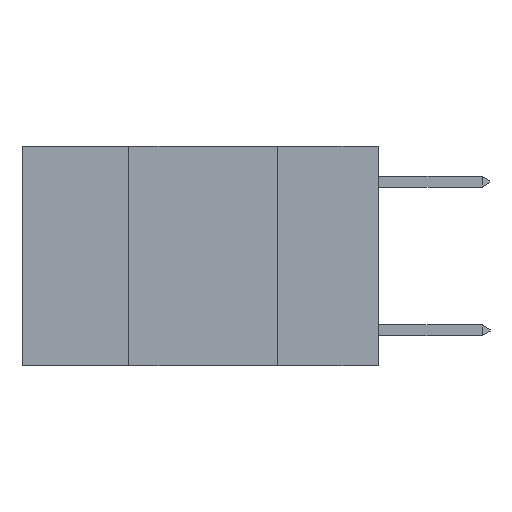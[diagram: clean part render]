
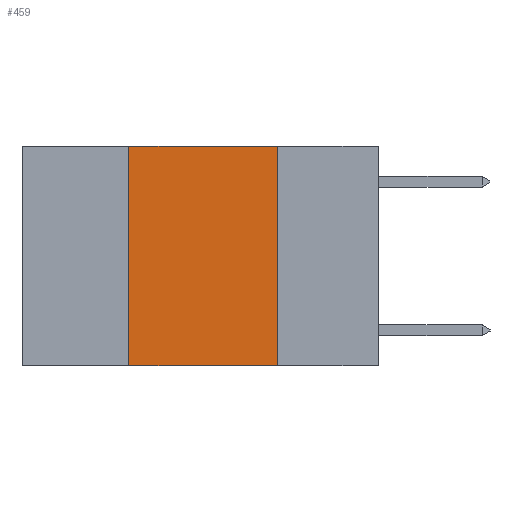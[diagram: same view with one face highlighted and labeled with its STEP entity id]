
A CAD part, left-side view. The second image highlights one B-rep face of the part: STEP entity #459.
In plain terms, the highlighted planar face has unit normal (-1, 0, 0).
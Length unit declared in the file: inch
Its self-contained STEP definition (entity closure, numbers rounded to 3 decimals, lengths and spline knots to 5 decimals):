
#457 = VERTEX_POINT ( 'NONE', #8114 ) ;
#459 = ADVANCED_FACE ( 'NONE', ( #5461 ), #3901, .F. ) ;
#482 = EDGE_LOOP ( 'NONE', ( #6296, #4374, #7703, #4807 ) ) ;
#633 = CARTESIAN_POINT ( 'NONE',  ( 0., 0.17, 0. ) ) ;
#1164 = LINE ( 'NONE', #4576, #6140 ) ;
#1240 = LINE ( 'NONE', #3805, #8051 ) ;
#1251 = DIRECTION ( 'NONE',  ( 0., -1., 0. ) ) ;
#1376 = EDGE_CURVE ( 'NONE', #5073, #457, #5447, .T. ) ;
#1477 = EDGE_CURVE ( 'NONE', #7250, #457, #1240, .T. ) ;
#2249 = VERTEX_POINT ( 'NONE', #5056 ) ;
#2732 = CARTESIAN_POINT ( 'NONE',  ( 0., 0.6, 0. ) ) ;
#2778 = CARTESIAN_POINT ( 'NONE',  ( 0., 0.42, 0. ) ) ;
#2965 = DIRECTION ( 'NONE',  ( 1., 0., 0. ) ) ;
#3805 = CARTESIAN_POINT ( 'NONE',  ( 0., 0.6, -0.37 ) ) ;
#3901 = PLANE ( 'NONE',  #8796 ) ;
#3967 = CARTESIAN_POINT ( 'NONE',  ( 0., 0.17, 0. ) ) ;
#4143 = VECTOR ( 'NONE', #6821, 39.37008 ) ;
#4344 = LINE ( 'NONE', #2778, #4143 ) ;
#4374 = ORIENTED_EDGE ( 'NONE', *, *, #8383, .F. ) ;
#4576 = CARTESIAN_POINT ( 'NONE',  ( 0., 0.6, 0. ) ) ;
#4617 = DIRECTION ( 'NONE',  ( 0., 0., -1. ) ) ;
#4807 = ORIENTED_EDGE ( 'NONE', *, *, #1477, .T. ) ;
#5056 = CARTESIAN_POINT ( 'NONE',  ( 0., 0.42, 0. ) ) ;
#5073 = VERTEX_POINT ( 'NONE', #3967 ) ;
#5447 = LINE ( 'NONE', #633, #7301 ) ;
#5461 = FACE_OUTER_BOUND ( 'NONE', #482, .T. ) ;
#6140 = VECTOR ( 'NONE', #6647, 39.37008 ) ;
#6296 = ORIENTED_EDGE ( 'NONE', *, *, #1376, .F. ) ;
#6546 = DIRECTION ( 'NONE',  ( 0., 0., -1. ) ) ;
#6647 = DIRECTION ( 'NONE',  ( 0., -1., 0. ) ) ;
#6821 = DIRECTION ( 'NONE',  ( 0., 0., 1. ) ) ;
#7250 = VERTEX_POINT ( 'NONE', #8668 ) ;
#7301 = VECTOR ( 'NONE', #4617, 39.37008 ) ;
#7495 = EDGE_CURVE ( 'NONE', #7250, #2249, #4344, .T. ) ;
#7703 = ORIENTED_EDGE ( 'NONE', *, *, #7495, .F. ) ;
#8051 = VECTOR ( 'NONE', #1251, 39.37008 ) ;
#8114 = CARTESIAN_POINT ( 'NONE',  ( 0., 0.17, -0.37 ) ) ;
#8383 = EDGE_CURVE ( 'NONE', #2249, #5073, #1164, .T. ) ;
#8668 = CARTESIAN_POINT ( 'NONE',  ( 0., 0.42, -0.37 ) ) ;
#8796 = AXIS2_PLACEMENT_3D ( 'NONE', #2732, #2965, #6546 ) ;
